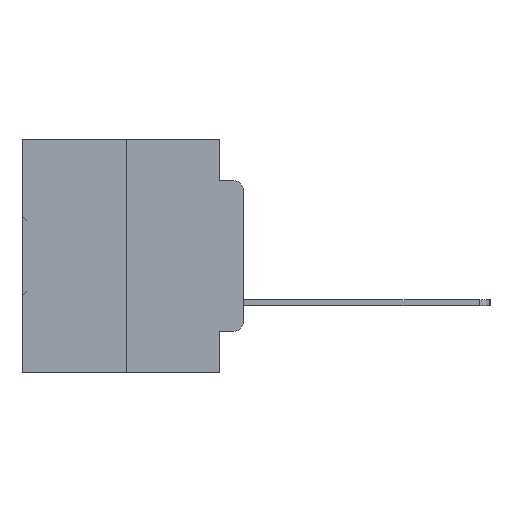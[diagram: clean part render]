
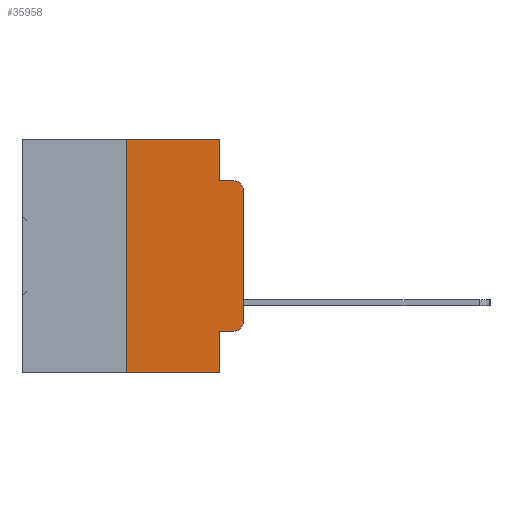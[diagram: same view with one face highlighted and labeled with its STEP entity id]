
A CAD part, left-side view. The second image highlights one B-rep face of the part: STEP entity #35958.
In plain terms, the highlighted planar face has unit normal (-1, 0, 0).
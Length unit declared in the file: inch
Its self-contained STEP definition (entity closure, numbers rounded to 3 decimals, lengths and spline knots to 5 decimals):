
#757 = VERTEX_POINT ( 'NONE', #17158 ) ;
#970 = DIRECTION ( 'NONE',  ( 0., 0., -1. ) ) ;
#1126 = VERTEX_POINT ( 'NONE', #33462 ) ;
#1333 = CIRCLE ( 'NONE', #1939, 0.02 ) ;
#1376 = CARTESIAN_POINT ( 'NONE',  ( 0., 0.051, 0. ) ) ;
#1939 = AXIS2_PLACEMENT_3D ( 'NONE', #33547, #16659, #36331 ) ;
#2743 = DIRECTION ( 'NONE',  ( 0., -1., 0. ) ) ;
#3363 = CARTESIAN_POINT ( 'NONE',  ( 0., 0.473, 0. ) ) ;
#3581 = AXIS2_PLACEMENT_3D ( 'NONE', #21000, #3810, #23851 ) ;
#3810 = DIRECTION ( 'NONE',  ( -1., 0., 0. ) ) ;
#4296 = DIRECTION ( 'NONE',  ( 0., 0., -1. ) ) ;
#4335 = VECTOR ( 'NONE', #19405, 39.37008 ) ;
#4765 = CARTESIAN_POINT ( 'NONE',  ( 0., 0.473, 0. ) ) ;
#5260 = LINE ( 'NONE', #10777, #4335 ) ;
#5418 = CARTESIAN_POINT ( 'NONE',  ( 0., 0.25, -0.5 ) ) ;
#6105 = LINE ( 'NONE', #3363, #35361 ) ;
#6193 = VERTEX_POINT ( 'NONE', #29418 ) ;
#6505 = EDGE_CURVE ( 'NONE', #30410, #22578, #1333, .T. ) ;
#7385 = VECTOR ( 'NONE', #970, 39.37008 ) ;
#7529 = PLANE ( 'NONE',  #22623 ) ;
#7561 = CARTESIAN_POINT ( 'NONE',  ( 0., 0.051, 0. ) ) ;
#7616 = VECTOR ( 'NONE', #32103, 39.37008 ) ;
#8937 = VECTOR ( 'NONE', #26235, 39.37008 ) ;
#10568 = DIRECTION ( 'NONE',  ( 1., 0., 0. ) ) ;
#10698 = DIRECTION ( 'NONE',  ( 0., -1., 0. ) ) ;
#10777 = CARTESIAN_POINT ( 'NONE',  ( 0., 0., 0. ) ) ;
#11406 = VECTOR ( 'NONE', #10698, 39.37008 ) ;
#12065 = DIRECTION ( 'NONE',  ( 0., -1., 0. ) ) ;
#12299 = LINE ( 'NONE', #19197, #11406 ) ;
#14678 = FACE_OUTER_BOUND ( 'NONE', #20972, .T. ) ;
#15009 = LINE ( 'NONE', #18238, #7385 ) ;
#15409 = ORIENTED_EDGE ( 'NONE', *, *, #21334, .F. ) ;
#15598 = CARTESIAN_POINT ( 'NONE',  ( 0., 0.25, 0. ) ) ;
#16659 = DIRECTION ( 'NONE',  ( -1., 0., 0. ) ) ;
#17068 = LINE ( 'NONE', #29287, #7616 ) ;
#17158 = CARTESIAN_POINT ( 'NONE',  ( 0., 0.051, -0.5 ) ) ;
#18120 = ORIENTED_EDGE ( 'NONE', *, *, #26028, .F. ) ;
#18238 = CARTESIAN_POINT ( 'NONE',  ( 0., 0.051, 0. ) ) ;
#18305 = VERTEX_POINT ( 'NONE', #26842 ) ;
#18359 = LINE ( 'NONE', #31766, #8937 ) ;
#18538 = ORIENTED_EDGE ( 'NONE', *, *, #6505, .T. ) ;
#19197 = CARTESIAN_POINT ( 'NONE',  ( 0., 0.051, -0.4115 ) ) ;
#19405 = DIRECTION ( 'NONE',  ( 0., 0., 1. ) ) ;
#19887 = EDGE_CURVE ( 'NONE', #6193, #1126, #12299, .T. ) ;
#20321 = CARTESIAN_POINT ( 'NONE',  ( 0., 0.051, -0.0885 ) ) ;
#20329 = ORIENTED_EDGE ( 'NONE', *, *, #33824, .F. ) ;
#20972 = EDGE_LOOP ( 'NONE', ( #25162, #18538, #20329, #27804, #29572, #15409, #22991, #18120, #35696, #30014 ) ) ;
#21000 = CARTESIAN_POINT ( 'NONE',  ( 0., 0.02, -0.3915 ) ) ;
#21334 = EDGE_CURVE ( 'NONE', #31280, #35360, #18359, .T. ) ;
#21657 = CIRCLE ( 'NONE', #3581, 0.02 ) ;
#22322 = EDGE_CURVE ( 'NONE', #18305, #30410, #5260, .T. ) ;
#22578 = VERTEX_POINT ( 'NONE', #34493 ) ;
#22623 = AXIS2_PLACEMENT_3D ( 'NONE', #4765, #10568, #30384 ) ;
#22991 = ORIENTED_EDGE ( 'NONE', *, *, #30805, .T. ) ;
#23024 = VERTEX_POINT ( 'NONE', #20321 ) ;
#23090 = EDGE_CURVE ( 'NONE', #35360, #27985, #6105, .T. ) ;
#23851 = DIRECTION ( 'NONE',  ( 0., 0., -1. ) ) ;
#24424 = EDGE_CURVE ( 'NONE', #27985, #23024, #15009, .T. ) ;
#25162 = ORIENTED_EDGE ( 'NONE', *, *, #22322, .T. ) ;
#26028 = EDGE_CURVE ( 'NONE', #6193, #757, #34322, .T. ) ;
#26235 = DIRECTION ( 'NONE',  ( 0., 0., 1. ) ) ;
#26842 = CARTESIAN_POINT ( 'NONE',  ( 0., 0., -0.3915 ) ) ;
#27804 = ORIENTED_EDGE ( 'NONE', *, *, #24424, .F. ) ;
#27985 = VERTEX_POINT ( 'NONE', #7561 ) ;
#29230 = CARTESIAN_POINT ( 'NONE',  ( 0., 0., -0.1085 ) ) ;
#29287 = CARTESIAN_POINT ( 'NONE',  ( 0., 0.051, -0.0885 ) ) ;
#29418 = CARTESIAN_POINT ( 'NONE',  ( 0., 0.051, -0.4115 ) ) ;
#29572 = ORIENTED_EDGE ( 'NONE', *, *, #23090, .F. ) ;
#30014 = ORIENTED_EDGE ( 'NONE', *, *, #32585, .T. ) ;
#30384 = DIRECTION ( 'NONE',  ( 0., 0., -1. ) ) ;
#30410 = VERTEX_POINT ( 'NONE', #29230 ) ;
#30805 = EDGE_CURVE ( 'NONE', #31280, #757, #32327, .T. ) ;
#31280 = VERTEX_POINT ( 'NONE', #5418 ) ;
#31438 = VECTOR ( 'NONE', #2743, 39.37008 ) ;
#31766 = CARTESIAN_POINT ( 'NONE',  ( 0., 0.25, 0. ) ) ;
#32103 = DIRECTION ( 'NONE',  ( 0., -1., 0. ) ) ;
#32327 = LINE ( 'NONE', #36759, #31438 ) ;
#32585 = EDGE_CURVE ( 'NONE', #1126, #18305, #21657, .T. ) ;
#33453 = VECTOR ( 'NONE', #4296, 39.37008 ) ;
#33462 = CARTESIAN_POINT ( 'NONE',  ( 0., 0.02, -0.4115 ) ) ;
#33547 = CARTESIAN_POINT ( 'NONE',  ( 0., 0.02, -0.1085 ) ) ;
#33824 = EDGE_CURVE ( 'NONE', #23024, #22578, #17068, .T. ) ;
#34322 = LINE ( 'NONE', #1376, #33453 ) ;
#34493 = CARTESIAN_POINT ( 'NONE',  ( 0., 0.02, -0.0885 ) ) ;
#35360 = VERTEX_POINT ( 'NONE', #15598 ) ;
#35361 = VECTOR ( 'NONE', #12065, 39.37008 ) ;
#35696 = ORIENTED_EDGE ( 'NONE', *, *, #19887, .T. ) ;
#35958 = ADVANCED_FACE ( 'NONE', ( #14678 ), #7529, .F. ) ;
#36331 = DIRECTION ( 'NONE',  ( 0., 0., -1. ) ) ;
#36759 = CARTESIAN_POINT ( 'NONE',  ( 0., 0.473, -0.5 ) ) ;
